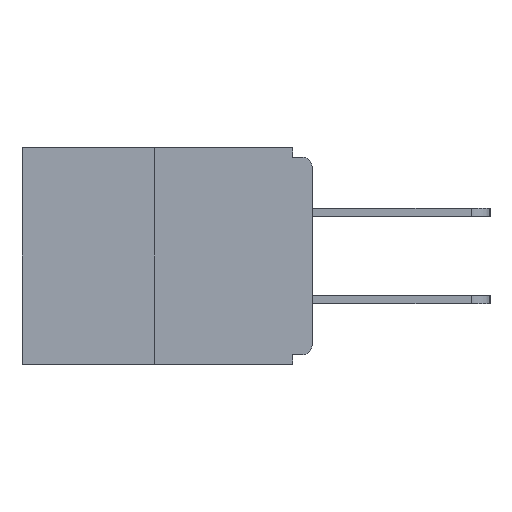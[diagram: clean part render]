
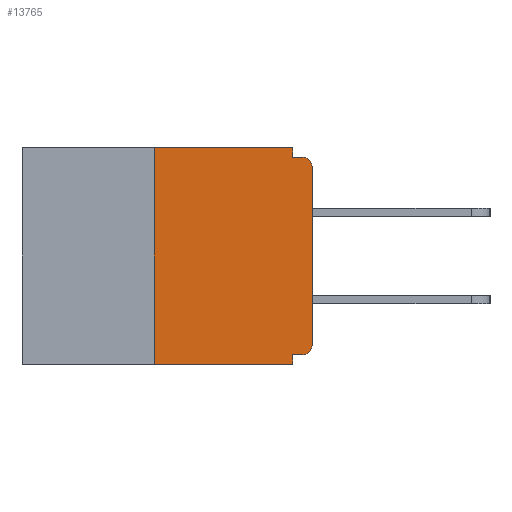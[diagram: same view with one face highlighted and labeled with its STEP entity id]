
A CAD part, left-side view. The second image highlights one B-rep face of the part: STEP entity #13765.
In plain terms, the highlighted planar face has unit normal (-1, 0, 0).
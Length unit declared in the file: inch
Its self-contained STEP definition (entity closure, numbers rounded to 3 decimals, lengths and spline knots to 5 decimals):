
#201 = ORIENTED_EDGE ( 'NONE', *, *, #2695, .T. ) ;
#418 = PLANE ( 'NONE',  #1347 ) ;
#456 = CARTESIAN_POINT ( 'NONE',  ( 0., 0.46, -0.343 ) ) ;
#468 = EDGE_LOOP ( 'NONE', ( #11912, #2055, #201, #13976, #1246, #13713, #4098, #7706, #12544, #13872 ) ) ;
#741 = DIRECTION ( 'NONE',  ( -1., 0., 0. ) ) ;
#771 = VECTOR ( 'NONE', #8777, 39.37008 ) ;
#772 = EDGE_CURVE ( 'NONE', #8468, #7997, #15260, .T. ) ;
#917 = VECTOR ( 'NONE', #14788, 39.37008 ) ;
#964 = VERTEX_POINT ( 'NONE', #12000 ) ;
#966 = LINE ( 'NONE', #2421, #1178 ) ;
#1038 = EDGE_CURVE ( 'NONE', #7997, #964, #966, .T. ) ;
#1178 = VECTOR ( 'NONE', #12232, 39.37008 ) ;
#1246 = ORIENTED_EDGE ( 'NONE', *, *, #8715, .F. ) ;
#1314 = VECTOR ( 'NONE', #15946, 39.37008 ) ;
#1347 = AXIS2_PLACEMENT_3D ( 'NONE', #2939, #7930, #14235 ) ;
#1369 = CARTESIAN_POINT ( 'NONE',  ( 0., 0., -0.328 ) ) ;
#1422 = CARTESIAN_POINT ( 'NONE',  ( 0., 0.031, 0. ) ) ;
#1458 = CARTESIAN_POINT ( 'NONE',  ( 0., 0.015, -0.328 ) ) ;
#2050 = VECTOR ( 'NONE', #3667, 39.37008 ) ;
#2055 = ORIENTED_EDGE ( 'NONE', *, *, #4585, .F. ) ;
#2161 = EDGE_CURVE ( 'NONE', #7861, #5512, #9779, .T. ) ;
#2421 = CARTESIAN_POINT ( 'NONE',  ( 0., 0.031, 0. ) ) ;
#2569 = DIRECTION ( 'NONE',  ( 0., -1., 0. ) ) ;
#2695 = EDGE_CURVE ( 'NONE', #14859, #5512, #15163, .T. ) ;
#2939 = CARTESIAN_POINT ( 'NONE',  ( 0., 0.46, 0. ) ) ;
#3667 = DIRECTION ( 'NONE',  ( 0., 1., 0. ) ) ;
#4098 = ORIENTED_EDGE ( 'NONE', *, *, #9186, .T. ) ;
#4151 = CIRCLE ( 'NONE', #13552, 0.015 ) ;
#4428 = EDGE_CURVE ( 'NONE', #13154, #15206, #6275, .T. ) ;
#4585 = EDGE_CURVE ( 'NONE', #14859, #8468, #8554, .T. ) ;
#4788 = DIRECTION ( 'NONE',  ( 0., 0., -1. ) ) ;
#5034 = LINE ( 'NONE', #9997, #771 ) ;
#5512 = VERTEX_POINT ( 'NONE', #9877 ) ;
#6006 = LINE ( 'NONE', #10982, #9397 ) ;
#6083 = CARTESIAN_POINT ( 'NONE',  ( 0., 0.031, -0.328 ) ) ;
#6227 = VECTOR ( 'NONE', #2569, 39.37008 ) ;
#6275 = CIRCLE ( 'NONE', #9389, 0.015 ) ;
#6428 = VECTOR ( 'NONE', #15028, 39.37008 ) ;
#6760 = CARTESIAN_POINT ( 'NONE',  ( 0., 0.25, -0.343 ) ) ;
#7240 = DIRECTION ( 'NONE',  ( -1., 0., 0. ) ) ;
#7472 = CARTESIAN_POINT ( 'NONE',  ( 0., 0.015, -0.313 ) ) ;
#7706 = ORIENTED_EDGE ( 'NONE', *, *, #4428, .T. ) ;
#7861 = VERTEX_POINT ( 'NONE', #6083 ) ;
#7878 = EDGE_CURVE ( 'NONE', #15850, #13088, #4151, .T. ) ;
#7930 = DIRECTION ( 'NONE',  ( 1., 0., 0. ) ) ;
#7997 = VERTEX_POINT ( 'NONE', #1422 ) ;
#8004 = DIRECTION ( 'NONE',  ( 0., 0., -1. ) ) ;
#8274 = CARTESIAN_POINT ( 'NONE',  ( 0., 0., -0.313 ) ) ;
#8468 = VERTEX_POINT ( 'NONE', #10280 ) ;
#8554 = LINE ( 'NONE', #13404, #1314 ) ;
#8715 = EDGE_CURVE ( 'NONE', #15850, #7861, #12572, .T. ) ;
#8777 = DIRECTION ( 'NONE',  ( 0., 0., 1. ) ) ;
#9186 = EDGE_CURVE ( 'NONE', #13088, #13154, #5034, .T. ) ;
#9389 = AXIS2_PLACEMENT_3D ( 'NONE', #13248, #741, #8004 ) ;
#9397 = VECTOR ( 'NONE', #15990, 39.37008 ) ;
#9779 = LINE ( 'NONE', #11261, #917 ) ;
#9877 = CARTESIAN_POINT ( 'NONE',  ( 0., 0.031, -0.343 ) ) ;
#9997 = CARTESIAN_POINT ( 'NONE',  ( 0., 0., 0. ) ) ;
#10157 = CARTESIAN_POINT ( 'NONE',  ( 0., 0.015, -0.015 ) ) ;
#10280 = CARTESIAN_POINT ( 'NONE',  ( 0., 0.25, 0. ) ) ;
#10632 = EDGE_CURVE ( 'NONE', #964, #15206, #6006, .T. ) ;
#10982 = CARTESIAN_POINT ( 'NONE',  ( 0., 0., -0.015 ) ) ;
#11261 = CARTESIAN_POINT ( 'NONE',  ( 0., 0.031, -0.343 ) ) ;
#11337 = CARTESIAN_POINT ( 'NONE',  ( 0., 0.46, 0. ) ) ;
#11601 = FACE_OUTER_BOUND ( 'NONE', #468, .T. ) ;
#11912 = ORIENTED_EDGE ( 'NONE', *, *, #772, .F. ) ;
#12000 = CARTESIAN_POINT ( 'NONE',  ( 0., 0.031, -0.015 ) ) ;
#12232 = DIRECTION ( 'NONE',  ( 0., 0., -1. ) ) ;
#12544 = ORIENTED_EDGE ( 'NONE', *, *, #10632, .F. ) ;
#12572 = LINE ( 'NONE', #1369, #2050 ) ;
#13088 = VERTEX_POINT ( 'NONE', #8274 ) ;
#13154 = VERTEX_POINT ( 'NONE', #15731 ) ;
#13248 = CARTESIAN_POINT ( 'NONE',  ( 0., 0.015, -0.03 ) ) ;
#13404 = CARTESIAN_POINT ( 'NONE',  ( 0., 0.25, 0. ) ) ;
#13552 = AXIS2_PLACEMENT_3D ( 'NONE', #7472, #7240, #4788 ) ;
#13713 = ORIENTED_EDGE ( 'NONE', *, *, #7878, .T. ) ;
#13765 = ADVANCED_FACE ( 'NONE', ( #11601 ), #418, .F. ) ;
#13872 = ORIENTED_EDGE ( 'NONE', *, *, #1038, .F. ) ;
#13976 = ORIENTED_EDGE ( 'NONE', *, *, #2161, .F. ) ;
#14235 = DIRECTION ( 'NONE',  ( 0., 0., -1. ) ) ;
#14788 = DIRECTION ( 'NONE',  ( 0., 0., -1. ) ) ;
#14859 = VERTEX_POINT ( 'NONE', #6760 ) ;
#15028 = DIRECTION ( 'NONE',  ( 0., -1., 0. ) ) ;
#15163 = LINE ( 'NONE', #456, #6227 ) ;
#15206 = VERTEX_POINT ( 'NONE', #10157 ) ;
#15260 = LINE ( 'NONE', #11337, #6428 ) ;
#15731 = CARTESIAN_POINT ( 'NONE',  ( 0., 0., -0.03 ) ) ;
#15850 = VERTEX_POINT ( 'NONE', #1458 ) ;
#15946 = DIRECTION ( 'NONE',  ( 0., 0., 1. ) ) ;
#15990 = DIRECTION ( 'NONE',  ( 0., -1., 0. ) ) ;
